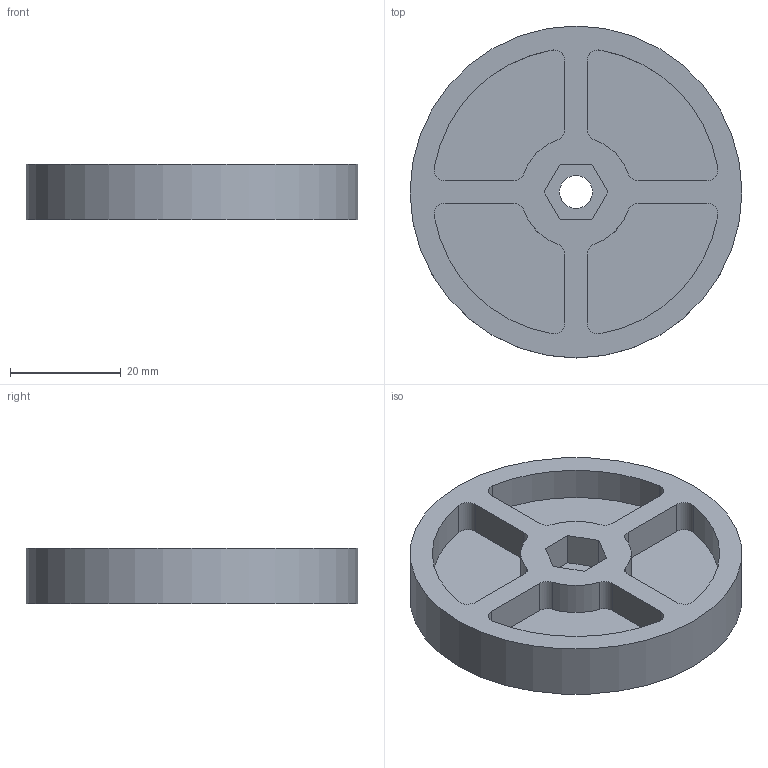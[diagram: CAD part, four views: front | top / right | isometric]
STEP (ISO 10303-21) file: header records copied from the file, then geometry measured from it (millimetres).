
FILE_DESCRIPTION((''),'2;1');
FILE_NAME('FittingTool1.stp','2015-10-05T00:24:00',('JamesRPatrick'),(''),'Autodesk Inventor 2012','Autodesk Inventor 2012','');
FILE_SCHEMA(('AUTOMOTIVE_DESIGN { 1 0 10303 214 1 1 1 1 }'));
Length unit declared in the file: millimetre
Products named in the file (1): FittingTool1
Bounding box: 60 x 60 x 10 mm (x, y, z)
Volume: 18400.3 mm3; surface area: 9629.5 mm2
Topology: 1 solids, 1 shells, 47 faces, 120 edges, 80 vertices
Faces by surface type: cylinder 26, plane 21
Full cylindrical faces by diameter (mm): 6 x1, 60 x1
Entity records: 1474 total; most frequent: DIRECTION 266, CARTESIAN_POINT 246, ORIENTED_EDGE 236, EDGE_CURVE 118, AXIS2_PLACEMENT_3D 100, VERTEX_POINT 80, VECTOR 66, LINE 66
